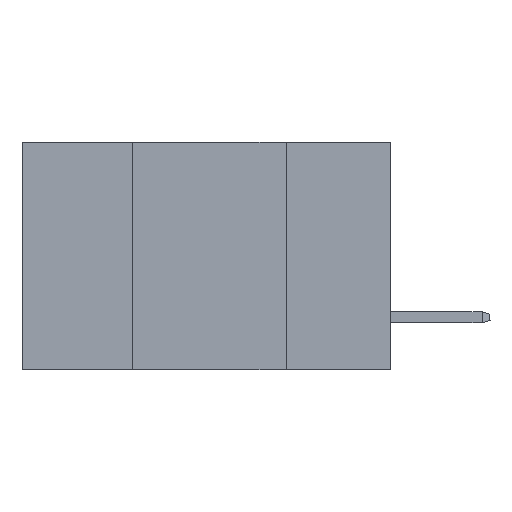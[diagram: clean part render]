
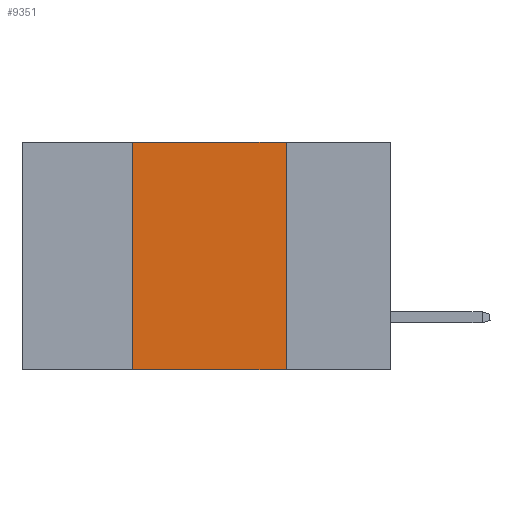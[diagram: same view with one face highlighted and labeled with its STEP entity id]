
A CAD part, left-side view. The second image highlights one B-rep face of the part: STEP entity #9351.
In plain terms, the highlighted planar face has unit normal (-1, 0, 0).
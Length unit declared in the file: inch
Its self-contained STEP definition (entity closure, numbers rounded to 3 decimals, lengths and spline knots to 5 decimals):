
#34 = ORIENTED_EDGE ( 'NONE', *, *, #22666, .F. ) ;
#727 = CARTESIAN_POINT ( 'NONE',  ( 0., 0.6, 0. ) ) ;
#837 = CARTESIAN_POINT ( 'NONE',  ( 0., 0.17, 0. ) ) ;
#2623 = VECTOR ( 'NONE', #31422, 39.37008 ) ;
#2881 = AXIS2_PLACEMENT_3D ( 'NONE', #11569, #3230, #9072 ) ;
#3230 = DIRECTION ( 'NONE',  ( 1., 0., 0. ) ) ;
#4005 = CARTESIAN_POINT ( 'NONE',  ( 0., 0.42, -0.37 ) ) ;
#5121 = ORIENTED_EDGE ( 'NONE', *, *, #18346, .F. ) ;
#5490 = ORIENTED_EDGE ( 'NONE', *, *, #36178, .F. ) ;
#6155 = CARTESIAN_POINT ( 'NONE',  ( 0., 0.17, 0. ) ) ;
#6626 = FACE_OUTER_BOUND ( 'NONE', #20118, .T. ) ;
#9072 = DIRECTION ( 'NONE',  ( 0., 0., -1. ) ) ;
#9351 = ADVANCED_FACE ( 'NONE', ( #6626 ), #14515, .F. ) ;
#10691 = LINE ( 'NONE', #16741, #25661 ) ;
#11462 = VERTEX_POINT ( 'NONE', #15152 ) ;
#11569 = CARTESIAN_POINT ( 'NONE',  ( 0., 0.6, 0. ) ) ;
#14515 = PLANE ( 'NONE',  #2881 ) ;
#15060 = VECTOR ( 'NONE', #31096, 39.37008 ) ;
#15152 = CARTESIAN_POINT ( 'NONE',  ( 0., 0.42, 0. ) ) ;
#15164 = ORIENTED_EDGE ( 'NONE', *, *, #22766, .T. ) ;
#16741 = CARTESIAN_POINT ( 'NONE',  ( 0., 0.42, 0. ) ) ;
#18346 = EDGE_CURVE ( 'NONE', #11462, #26560, #35888, .T. ) ;
#19454 = VECTOR ( 'NONE', #31465, 39.37008 ) ;
#20118 = EDGE_LOOP ( 'NONE', ( #5490, #5121, #34, #15164 ) ) ;
#20556 = DIRECTION ( 'NONE',  ( 0., 0., 1. ) ) ;
#20826 = LINE ( 'NONE', #25733, #15060 ) ;
#22666 = EDGE_CURVE ( 'NONE', #25772, #11462, #10691, .T. ) ;
#22766 = EDGE_CURVE ( 'NONE', #25772, #36187, #20826, .T. ) ;
#24794 = LINE ( 'NONE', #6155, #2623 ) ;
#25661 = VECTOR ( 'NONE', #20556, 39.37008 ) ;
#25733 = CARTESIAN_POINT ( 'NONE',  ( 0., 0.6, -0.37 ) ) ;
#25772 = VERTEX_POINT ( 'NONE', #4005 ) ;
#26560 = VERTEX_POINT ( 'NONE', #837 ) ;
#31096 = DIRECTION ( 'NONE',  ( 0., -1., 0. ) ) ;
#31422 = DIRECTION ( 'NONE',  ( 0., 0., -1. ) ) ;
#31465 = DIRECTION ( 'NONE',  ( 0., -1., 0. ) ) ;
#31532 = CARTESIAN_POINT ( 'NONE',  ( 0., 0.17, -0.37 ) ) ;
#35888 = LINE ( 'NONE', #727, #19454 ) ;
#36178 = EDGE_CURVE ( 'NONE', #26560, #36187, #24794, .T. ) ;
#36187 = VERTEX_POINT ( 'NONE', #31532 ) ;
